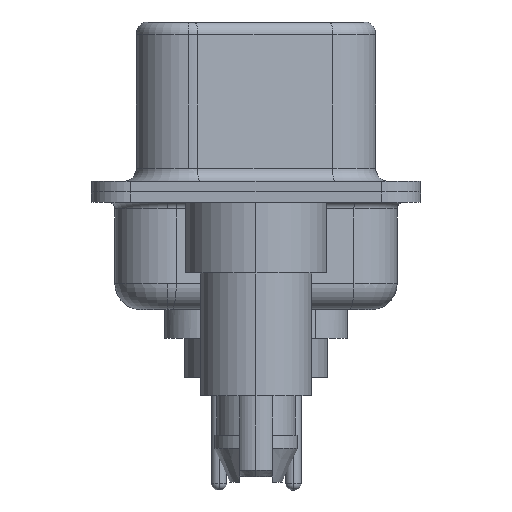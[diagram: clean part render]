
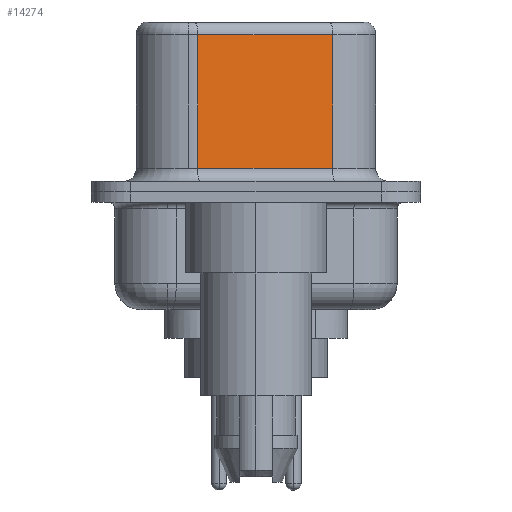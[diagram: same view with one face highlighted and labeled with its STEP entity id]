
A CAD part, left-side view. The second image highlights one B-rep face of the part: STEP entity #14274.
In plain terms, the highlighted planar face has unit normal (-0.985, -0.174, 0).
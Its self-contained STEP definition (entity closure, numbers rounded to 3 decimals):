
#832 = CARTESIAN_POINT ( 'NONE',  ( 4.585, -2.927, 6.52 ) ) ;
#952 = FACE_OUTER_BOUND ( 'NONE', #11543, .T. ) ;
#981 = VECTOR ( 'NONE', #7274, 1000. ) ;
#1371 = ORIENTED_EDGE ( 'NONE', *, *, #19051, .T. ) ;
#3026 = EDGE_CURVE ( 'NONE', #18575, #12971, #3383, .T. ) ;
#3383 = LINE ( 'NONE', #10131, #14707 ) ;
#3723 = VERTEX_POINT ( 'NONE', #19122 ) ;
#3963 = CARTESIAN_POINT ( 'NONE',  ( 4.585, -2.927, 6.52 ) ) ;
#5004 = EDGE_CURVE ( 'NONE', #18575, #19115, #17896, .T. ) ;
#5304 = DIRECTION ( 'NONE',  ( 0.985, 0.174, 0. ) ) ;
#5693 = DIRECTION ( 'NONE',  ( -0.174, 0.985, 0. ) ) ;
#5710 = CARTESIAN_POINT ( 'NONE',  ( 3.675, 2.233, 6.52 ) ) ;
#5760 = CARTESIAN_POINT ( 'NONE',  ( 4.585, -2.927, 0.9 ) ) ;
#6016 = CARTESIAN_POINT ( 'NONE',  ( 3.675, 2.233, 6.02 ) ) ;
#6150 = CARTESIAN_POINT ( 'NONE',  ( 4.585, -2.927, 6.02 ) ) ;
#7274 = DIRECTION ( 'NONE',  ( 0.174, -0.985, 0. ) ) ;
#8412 = LINE ( 'NONE', #5760, #981 ) ;
#9525 = ORIENTED_EDGE ( 'NONE', *, *, #5004, .F. ) ;
#9904 = AXIS2_PLACEMENT_3D ( 'NONE', #832, #5304, #15686 ) ;
#10131 = CARTESIAN_POINT ( 'NONE',  ( 4.585, -2.927, 6.02 ) ) ;
#10253 = LINE ( 'NONE', #5710, #17658 ) ;
#10257 = ORIENTED_EDGE ( 'NONE', *, *, #3026, .T. ) ;
#11119 = EDGE_CURVE ( 'NONE', #3723, #19115, #8412, .T. ) ;
#11543 = EDGE_LOOP ( 'NONE', ( #9525, #10257, #1371, #13396 ) ) ;
#12971 = VERTEX_POINT ( 'NONE', #6016 ) ;
#13396 = ORIENTED_EDGE ( 'NONE', *, *, #11119, .T. ) ;
#13959 = VECTOR ( 'NONE', #17503, 1000. ) ;
#14274 = ADVANCED_FACE ( 'NONE', ( #952 ), #18611, .F. ) ;
#14477 = CARTESIAN_POINT ( 'NONE',  ( 4.585, -2.927, 0.9 ) ) ;
#14598 = DIRECTION ( 'NONE',  ( 0., 0., -1. ) ) ;
#14707 = VECTOR ( 'NONE', #5693, 1000. ) ;
#15686 = DIRECTION ( 'NONE',  ( -0.174, 0.985, 0. ) ) ;
#17503 = DIRECTION ( 'NONE',  ( 0., 0., -1. ) ) ;
#17658 = VECTOR ( 'NONE', #14598, 1000. ) ;
#17896 = LINE ( 'NONE', #3963, #13959 ) ;
#18575 = VERTEX_POINT ( 'NONE', #6150 ) ;
#18611 = PLANE ( 'NONE',  #9904 ) ;
#19051 = EDGE_CURVE ( 'NONE', #12971, #3723, #10253, .T. ) ;
#19115 = VERTEX_POINT ( 'NONE', #14477 ) ;
#19122 = CARTESIAN_POINT ( 'NONE',  ( 3.675, 2.233, 0.9 ) ) ;
